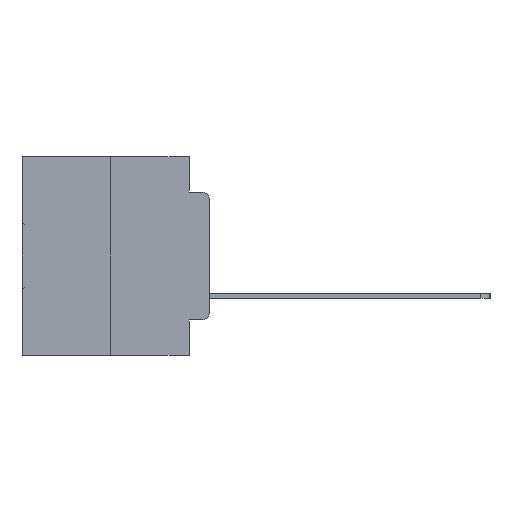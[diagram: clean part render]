
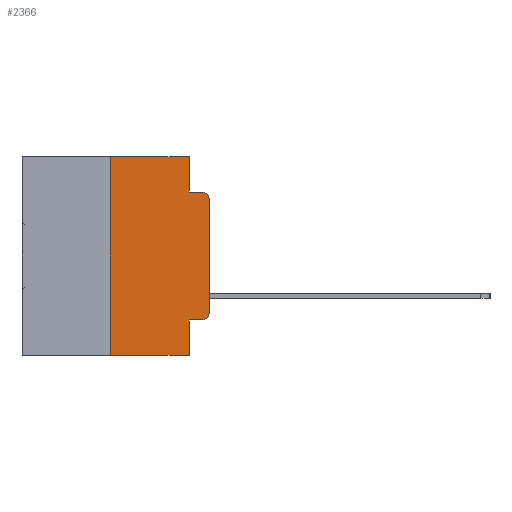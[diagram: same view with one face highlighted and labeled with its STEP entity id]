
A CAD part, left-side view. The second image highlights one B-rep face of the part: STEP entity #2366.
In plain terms, the highlighted planar face has unit normal (-1, 0, 0).
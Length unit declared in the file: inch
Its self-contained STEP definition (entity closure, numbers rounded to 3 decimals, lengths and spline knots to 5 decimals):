
#145 = CARTESIAN_POINT ( 'NONE',  ( 0., 0.02, -0.0885 ) ) ;
#1246 = CARTESIAN_POINT ( 'NONE',  ( 0., 0.25, 0. ) ) ;
#1342 = ORIENTED_EDGE ( 'NONE', *, *, #25945, .T. ) ;
#1448 = VERTEX_POINT ( 'NONE', #145 ) ;
#1821 = LINE ( 'NONE', #14801, #26311 ) ;
#2366 = ADVANCED_FACE ( 'NONE', ( #17116 ), #18148, .F. ) ;
#2639 = VERTEX_POINT ( 'NONE', #9145 ) ;
#2698 = EDGE_CURVE ( 'NONE', #29804, #15041, #1821, .T. ) ;
#2703 = CARTESIAN_POINT ( 'NONE',  ( 0., 0., -0.3915 ) ) ;
#2771 = CARTESIAN_POINT ( 'NONE',  ( 0., 0.051, -0.4115 ) ) ;
#3261 = CARTESIAN_POINT ( 'NONE',  ( 0., 0.051, -0.0885 ) ) ;
#4424 = VECTOR ( 'NONE', #17277, 39.37008 ) ;
#4673 = ORIENTED_EDGE ( 'NONE', *, *, #23784, .T. ) ;
#4755 = AXIS2_PLACEMENT_3D ( 'NONE', #24674, #10525, #27034 ) ;
#5118 = ORIENTED_EDGE ( 'NONE', *, *, #2698, .F. ) ;
#5330 = CARTESIAN_POINT ( 'NONE',  ( 0., 0.051, 0. ) ) ;
#5426 = LINE ( 'NONE', #25811, #11753 ) ;
#5906 = AXIS2_PLACEMENT_3D ( 'NONE', #24867, #10716, #27221 ) ;
#7625 = CARTESIAN_POINT ( 'NONE',  ( 0., 0., -0.1085 ) ) ;
#7906 = ORIENTED_EDGE ( 'NONE', *, *, #28209, .F. ) ;
#8430 = VECTOR ( 'NONE', #28156, 39.37008 ) ;
#8764 = VERTEX_POINT ( 'NONE', #20024 ) ;
#8856 = VECTOR ( 'NONE', #16901, 39.37008 ) ;
#8916 = EDGE_LOOP ( 'NONE', ( #17663, #29000, #7906, #17406, #26292, #5118, #27246, #10691, #4673, #1342 ) ) ;
#8983 = EDGE_CURVE ( 'NONE', #15041, #11907, #12071, .T. ) ;
#9145 = CARTESIAN_POINT ( 'NONE',  ( 0., 0.02, -0.4115 ) ) ;
#9172 = LINE ( 'NONE', #25822, #8430 ) ;
#9848 = CARTESIAN_POINT ( 'NONE',  ( 0., 0.25, -0.5 ) ) ;
#9882 = LINE ( 'NONE', #27330, #17667 ) ;
#10450 = VERTEX_POINT ( 'NONE', #2703 ) ;
#10525 = DIRECTION ( 'NONE',  ( -1., 0., 0. ) ) ;
#10691 = ORIENTED_EDGE ( 'NONE', *, *, #23371, .F. ) ;
#10716 = DIRECTION ( 'NONE',  ( -1., 0., 0. ) ) ;
#10783 = LINE ( 'NONE', #5330, #4424 ) ;
#11213 = VERTEX_POINT ( 'NONE', #29596 ) ;
#11673 = DIRECTION ( 'NONE',  ( 0., -1., 0. ) ) ;
#11753 = VECTOR ( 'NONE', #11673, 39.37008 ) ;
#11907 = VERTEX_POINT ( 'NONE', #30353 ) ;
#12071 = LINE ( 'NONE', #30128, #30045 ) ;
#12154 = CIRCLE ( 'NONE', #4755, 0.02 ) ;
#14219 = DIRECTION ( 'NONE',  ( 0., 0., -1. ) ) ;
#14255 = DIRECTION ( 'NONE',  ( 1., 0., 0. ) ) ;
#14656 = DIRECTION ( 'NONE',  ( 0., -1., 0. ) ) ;
#14801 = CARTESIAN_POINT ( 'NONE',  ( 0., 0.25, 0. ) ) ;
#15041 = VERTEX_POINT ( 'NONE', #1246 ) ;
#16249 = CARTESIAN_POINT ( 'NONE',  ( 0., 0.473, 0. ) ) ;
#16455 = DIRECTION ( 'NONE',  ( 0., 0., 1. ) ) ;
#16901 = DIRECTION ( 'NONE',  ( 0., -1., 0. ) ) ;
#17116 = FACE_OUTER_BOUND ( 'NONE', #8916, .T. ) ;
#17117 = AXIS2_PLACEMENT_3D ( 'NONE', #16249, #14255, #14219 ) ;
#17277 = DIRECTION ( 'NONE',  ( 0., 0., -1. ) ) ;
#17406 = ORIENTED_EDGE ( 'NONE', *, *, #27117, .F. ) ;
#17663 = ORIENTED_EDGE ( 'NONE', *, *, #22945, .T. ) ;
#17667 = VECTOR ( 'NONE', #29617, 39.37008 ) ;
#18148 = PLANE ( 'NONE',  #17117 ) ;
#19201 = VERTEX_POINT ( 'NONE', #7625 ) ;
#19242 = CARTESIAN_POINT ( 'NONE',  ( 0., 0.051, -0.0885 ) ) ;
#20024 = CARTESIAN_POINT ( 'NONE',  ( 0., 0.051, -0.5 ) ) ;
#20846 = DIRECTION ( 'NONE',  ( 0., -1., 0. ) ) ;
#22945 = EDGE_CURVE ( 'NONE', #10450, #19201, #9172, .T. ) ;
#23371 = EDGE_CURVE ( 'NONE', #11213, #8764, #9882, .T. ) ;
#23516 = VECTOR ( 'NONE', #14656, 39.37008 ) ;
#23784 = EDGE_CURVE ( 'NONE', #11213, #2639, #25002, .T. ) ;
#24674 = CARTESIAN_POINT ( 'NONE',  ( 0., 0.02, -0.1085 ) ) ;
#24867 = CARTESIAN_POINT ( 'NONE',  ( 0., 0.02, -0.3915 ) ) ;
#25002 = LINE ( 'NONE', #2771, #23516 ) ;
#25260 = CIRCLE ( 'NONE', #5906, 0.02 ) ;
#25811 = CARTESIAN_POINT ( 'NONE',  ( 0., 0.473, -0.5 ) ) ;
#25822 = CARTESIAN_POINT ( 'NONE',  ( 0., 0., 0. ) ) ;
#25945 = EDGE_CURVE ( 'NONE', #2639, #10450, #25260, .T. ) ;
#26292 = ORIENTED_EDGE ( 'NONE', *, *, #8983, .F. ) ;
#26311 = VECTOR ( 'NONE', #16455, 39.37008 ) ;
#27034 = DIRECTION ( 'NONE',  ( 0., 0., -1. ) ) ;
#27117 = EDGE_CURVE ( 'NONE', #11907, #28361, #10783, .T. ) ;
#27221 = DIRECTION ( 'NONE',  ( 0., 0., -1. ) ) ;
#27246 = ORIENTED_EDGE ( 'NONE', *, *, #30300, .T. ) ;
#27330 = CARTESIAN_POINT ( 'NONE',  ( 0., 0.051, 0. ) ) ;
#27657 = LINE ( 'NONE', #19242, #8856 ) ;
#28156 = DIRECTION ( 'NONE',  ( 0., 0., 1. ) ) ;
#28209 = EDGE_CURVE ( 'NONE', #28361, #1448, #27657, .T. ) ;
#28361 = VERTEX_POINT ( 'NONE', #3261 ) ;
#28818 = EDGE_CURVE ( 'NONE', #19201, #1448, #12154, .T. ) ;
#29000 = ORIENTED_EDGE ( 'NONE', *, *, #28818, .T. ) ;
#29596 = CARTESIAN_POINT ( 'NONE',  ( 0., 0.051, -0.4115 ) ) ;
#29617 = DIRECTION ( 'NONE',  ( 0., 0., -1. ) ) ;
#29804 = VERTEX_POINT ( 'NONE', #9848 ) ;
#30045 = VECTOR ( 'NONE', #20846, 39.37008 ) ;
#30128 = CARTESIAN_POINT ( 'NONE',  ( 0., 0.473, 0. ) ) ;
#30300 = EDGE_CURVE ( 'NONE', #29804, #8764, #5426, .T. ) ;
#30353 = CARTESIAN_POINT ( 'NONE',  ( 0., 0.051, 0. ) ) ;
